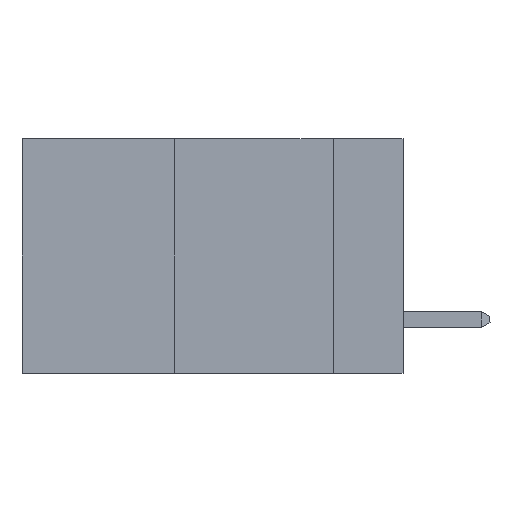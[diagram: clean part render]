
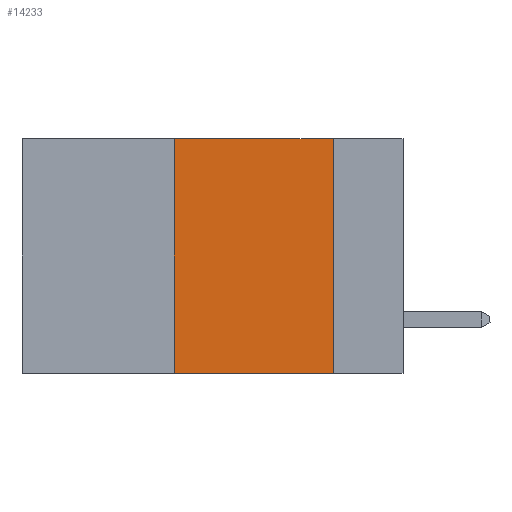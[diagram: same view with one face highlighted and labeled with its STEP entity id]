
A CAD part, left-side view. The second image highlights one B-rep face of the part: STEP entity #14233.
In plain terms, the highlighted planar face has unit normal (-1, 0, 0).
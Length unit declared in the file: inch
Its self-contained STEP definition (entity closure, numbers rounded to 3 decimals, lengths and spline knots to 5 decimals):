
#693 = EDGE_CURVE ( 'NONE', #1042, #7447, #7842, .T. ) ;
#762 = CARTESIAN_POINT ( 'NONE',  ( 0., 0.36, 0. ) ) ;
#1042 = VERTEX_POINT ( 'NONE', #10056 ) ;
#1475 = VERTEX_POINT ( 'NONE', #5783 ) ;
#2107 = DIRECTION ( 'NONE',  ( 0., 0., 1. ) ) ;
#2165 = DIRECTION ( 'NONE',  ( 1., 0., 0. ) ) ;
#2900 = VERTEX_POINT ( 'NONE', #3323 ) ;
#3238 = CARTESIAN_POINT ( 'NONE',  ( 0., 0.11, 0. ) ) ;
#3323 = CARTESIAN_POINT ( 'NONE',  ( 0., 0.36, -0.37 ) ) ;
#3681 = EDGE_LOOP ( 'NONE', ( #11316, #11692, #14999, #15401 ) ) ;
#3919 = VECTOR ( 'NONE', #7909, 39.37008 ) ;
#3951 = EDGE_CURVE ( 'NONE', #2900, #7447, #12015, .T. ) ;
#5783 = CARTESIAN_POINT ( 'NONE',  ( 0., 0.36, 0. ) ) ;
#6414 = LINE ( 'NONE', #762, #12795 ) ;
#6930 = AXIS2_PLACEMENT_3D ( 'NONE', #10196, #2165, #11420 ) ;
#7380 = CARTESIAN_POINT ( 'NONE',  ( 0., 0.11, -0.37 ) ) ;
#7447 = VERTEX_POINT ( 'NONE', #7380 ) ;
#7842 = LINE ( 'NONE', #3238, #10835 ) ;
#7909 = DIRECTION ( 'NONE',  ( 0., -1., 0. ) ) ;
#8905 = DIRECTION ( 'NONE',  ( 0., 0., -1. ) ) ;
#8988 = EDGE_CURVE ( 'NONE', #1475, #1042, #14207, .T. ) ;
#9825 = FACE_OUTER_BOUND ( 'NONE', #3681, .T. ) ;
#10056 = CARTESIAN_POINT ( 'NONE',  ( 0., 0.11, 0. ) ) ;
#10196 = CARTESIAN_POINT ( 'NONE',  ( 0., 0.6, 0. ) ) ;
#10835 = VECTOR ( 'NONE', #8905, 39.37008 ) ;
#11254 = VECTOR ( 'NONE', #16852, 39.37008 ) ;
#11316 = ORIENTED_EDGE ( 'NONE', *, *, #693, .F. ) ;
#11420 = DIRECTION ( 'NONE',  ( 0., 0., -1. ) ) ;
#11482 = CARTESIAN_POINT ( 'NONE',  ( 0., 0.6, -0.37 ) ) ;
#11692 = ORIENTED_EDGE ( 'NONE', *, *, #8988, .F. ) ;
#12015 = LINE ( 'NONE', #11482, #11254 ) ;
#12795 = VECTOR ( 'NONE', #2107, 39.37008 ) ;
#14174 = CARTESIAN_POINT ( 'NONE',  ( 0., 0.6, 0. ) ) ;
#14207 = LINE ( 'NONE', #14174, #3919 ) ;
#14233 = ADVANCED_FACE ( 'NONE', ( #9825 ), #15115, .F. ) ;
#14999 = ORIENTED_EDGE ( 'NONE', *, *, #16019, .F. ) ;
#15115 = PLANE ( 'NONE',  #6930 ) ;
#15401 = ORIENTED_EDGE ( 'NONE', *, *, #3951, .T. ) ;
#16019 = EDGE_CURVE ( 'NONE', #2900, #1475, #6414, .T. ) ;
#16852 = DIRECTION ( 'NONE',  ( 0., -1., 0. ) ) ;
